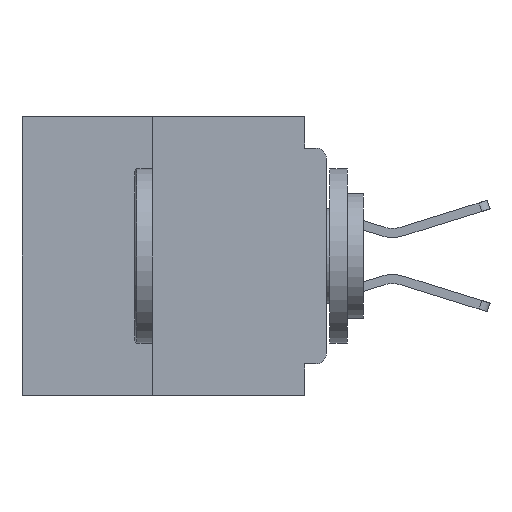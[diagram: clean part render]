
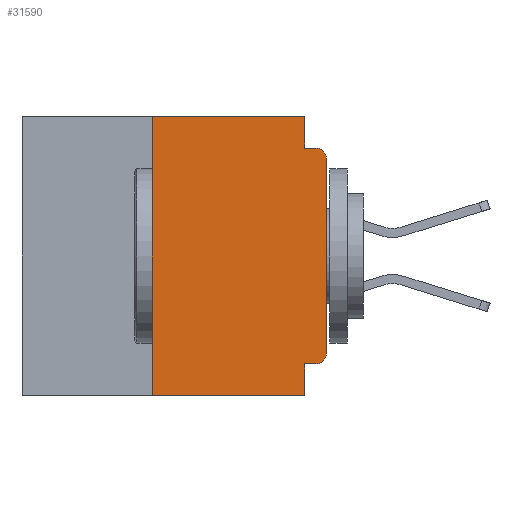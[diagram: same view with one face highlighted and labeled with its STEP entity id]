
A CAD part, left-side view. The second image highlights one B-rep face of the part: STEP entity #31590.
In plain terms, the highlighted planar face has unit normal (-1, 0, 0).
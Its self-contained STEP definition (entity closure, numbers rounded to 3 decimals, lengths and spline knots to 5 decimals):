
#134 = DIRECTION ( 'NONE',  ( 0., 0., -1. ) ) ;
#167 = LINE ( 'NONE', #49163, #48025 ) ;
#2944 = DIRECTION ( 'NONE',  ( 0., 0., -1. ) ) ;
#3805 = DIRECTION ( 'NONE',  ( 0., 0., -1. ) ) ;
#4819 = ORIENTED_EDGE ( 'NONE', *, *, #7803, .T. ) ;
#5775 = CARTESIAN_POINT ( 'NONE',  ( 0., 0., 0. ) ) ;
#5936 = LINE ( 'NONE', #54276, #18625 ) ;
#6459 = CARTESIAN_POINT ( 'NONE',  ( 0., 0., -0.06 ) ) ;
#7596 = VERTEX_POINT ( 'NONE', #22908 ) ;
#7803 = EDGE_CURVE ( 'NONE', #50664, #33889, #31660, .T. ) ;
#8249 = VECTOR ( 'NONE', #53485, 39.37008 ) ;
#10193 = VERTEX_POINT ( 'NONE', #15095 ) ;
#10473 = FACE_OUTER_BOUND ( 'NONE', #39620, .T. ) ;
#10834 = VECTOR ( 'NONE', #36608, 39.37008 ) ;
#14037 = VERTEX_POINT ( 'NONE', #52825 ) ;
#14038 = VECTOR ( 'NONE', #58044, 39.37008 ) ;
#14109 = DIRECTION ( 'NONE',  ( -1., 0., 0. ) ) ;
#14757 = VERTEX_POINT ( 'NONE', #58318 ) ;
#14826 = VERTEX_POINT ( 'NONE', #6459 ) ;
#15095 = CARTESIAN_POINT ( 'NONE',  ( 0., 0.015, -0.045 ) ) ;
#15217 = EDGE_CURVE ( 'NONE', #14826, #10193, #20259, .T. ) ;
#15760 = DIRECTION ( 'NONE',  ( 0., -1., 0. ) ) ;
#18625 = VECTOR ( 'NONE', #35677, 39.37008 ) ;
#20004 = CARTESIAN_POINT ( 'NONE',  ( 0., 0., -0.045 ) ) ;
#20259 = CIRCLE ( 'NONE', #28420, 0.015 ) ;
#20455 = VECTOR ( 'NONE', #44018, 39.37008 ) ;
#20880 = LINE ( 'NONE', #26800, #32079 ) ;
#22908 = CARTESIAN_POINT ( 'NONE',  ( 0., 0.015, -0.355 ) ) ;
#23308 = ORIENTED_EDGE ( 'NONE', *, *, #40323, .F. ) ;
#23654 = EDGE_CURVE ( 'NONE', #7596, #14757, #50395, .T. ) ;
#23836 = ORIENTED_EDGE ( 'NONE', *, *, #23654, .F. ) ;
#25021 = CARTESIAN_POINT ( 'NONE',  ( 0., 0.437, -0.4 ) ) ;
#26439 = DIRECTION ( 'NONE',  ( 1., 0., 0. ) ) ;
#26481 = AXIS2_PLACEMENT_3D ( 'NONE', #40672, #26439, #59667 ) ;
#26796 = LINE ( 'NONE', #20004, #14038 ) ;
#26800 = CARTESIAN_POINT ( 'NONE',  ( 0., 0.031, -0.4 ) ) ;
#26834 = EDGE_CURVE ( 'NONE', #50664, #54660, #5936, .T. ) ;
#27673 = ORIENTED_EDGE ( 'NONE', *, *, #26834, .F. ) ;
#28420 = AXIS2_PLACEMENT_3D ( 'NONE', #42783, #14109, #47535 ) ;
#28517 = AXIS2_PLACEMENT_3D ( 'NONE', #57260, #28807, #134 ) ;
#28807 = DIRECTION ( 'NONE',  ( -1., 0., 0. ) ) ;
#30177 = CARTESIAN_POINT ( 'NONE',  ( 0., 0.031, -0.4 ) ) ;
#31411 = EDGE_CURVE ( 'NONE', #34546, #14826, #58930, .T. ) ;
#31590 = ADVANCED_FACE ( 'NONE', ( #10473 ), #54910, .F. ) ;
#31660 = LINE ( 'NONE', #25021, #20455 ) ;
#31781 = CARTESIAN_POINT ( 'NONE',  ( 0., 0., -0.355 ) ) ;
#32079 = VECTOR ( 'NONE', #2944, 39.37008 ) ;
#32105 = ORIENTED_EDGE ( 'NONE', *, *, #38261, .F. ) ;
#32231 = ORIENTED_EDGE ( 'NONE', *, *, #60220, .T. ) ;
#33188 = CARTESIAN_POINT ( 'NONE',  ( 0., 0., -0.34 ) ) ;
#33889 = VERTEX_POINT ( 'NONE', #30177 ) ;
#34175 = CIRCLE ( 'NONE', #28517, 0.015 ) ;
#34546 = VERTEX_POINT ( 'NONE', #33188 ) ;
#34782 = EDGE_CURVE ( 'NONE', #54660, #14037, #167, .T. ) ;
#35677 = DIRECTION ( 'NONE',  ( 0., 0., 1. ) ) ;
#36435 = ORIENTED_EDGE ( 'NONE', *, *, #31411, .T. ) ;
#36608 = DIRECTION ( 'NONE',  ( 0., 1., 0. ) ) ;
#36715 = ORIENTED_EDGE ( 'NONE', *, *, #34782, .F. ) ;
#37222 = EDGE_CURVE ( 'NONE', #14757, #33889, #20880, .T. ) ;
#38261 = EDGE_CURVE ( 'NONE', #45914, #10193, #26796, .T. ) ;
#38738 = CARTESIAN_POINT ( 'NONE',  ( 0., 0.25, -0.4 ) ) ;
#39620 = EDGE_LOOP ( 'NONE', ( #36435, #57148, #32105, #23308, #36715, #27673, #4819, #41605, #23836, #32231 ) ) ;
#40323 = EDGE_CURVE ( 'NONE', #14037, #45914, #60676, .T. ) ;
#40672 = CARTESIAN_POINT ( 'NONE',  ( 0., 0.437, 0. ) ) ;
#41605 = ORIENTED_EDGE ( 'NONE', *, *, #37222, .F. ) ;
#42783 = CARTESIAN_POINT ( 'NONE',  ( 0., 0.015, -0.06 ) ) ;
#44018 = DIRECTION ( 'NONE',  ( 0., -1., 0. ) ) ;
#45914 = VERTEX_POINT ( 'NONE', #59237 ) ;
#46657 = VECTOR ( 'NONE', #3805, 39.37008 ) ;
#47535 = DIRECTION ( 'NONE',  ( 0., 0., -1. ) ) ;
#48025 = VECTOR ( 'NONE', #15760, 39.37008 ) ;
#49163 = CARTESIAN_POINT ( 'NONE',  ( 0., 0.437, 0. ) ) ;
#50395 = LINE ( 'NONE', #31781, #10834 ) ;
#50664 = VERTEX_POINT ( 'NONE', #38738 ) ;
#51380 = CARTESIAN_POINT ( 'NONE',  ( 0., 0.031, 0. ) ) ;
#52825 = CARTESIAN_POINT ( 'NONE',  ( 0., 0.031, 0. ) ) ;
#53485 = DIRECTION ( 'NONE',  ( 0., 0., 1. ) ) ;
#54276 = CARTESIAN_POINT ( 'NONE',  ( 0., 0.25, -0.4 ) ) ;
#54660 = VERTEX_POINT ( 'NONE', #60538 ) ;
#54910 = PLANE ( 'NONE',  #26481 ) ;
#57148 = ORIENTED_EDGE ( 'NONE', *, *, #15217, .T. ) ;
#57260 = CARTESIAN_POINT ( 'NONE',  ( 0., 0.015, -0.34 ) ) ;
#58044 = DIRECTION ( 'NONE',  ( 0., -1., 0. ) ) ;
#58318 = CARTESIAN_POINT ( 'NONE',  ( 0., 0.031, -0.355 ) ) ;
#58930 = LINE ( 'NONE', #5775, #8249 ) ;
#59237 = CARTESIAN_POINT ( 'NONE',  ( 0., 0.031, -0.045 ) ) ;
#59667 = DIRECTION ( 'NONE',  ( 0., 0., -1. ) ) ;
#60220 = EDGE_CURVE ( 'NONE', #7596, #34546, #34175, .T. ) ;
#60538 = CARTESIAN_POINT ( 'NONE',  ( 0., 0.25, 0. ) ) ;
#60676 = LINE ( 'NONE', #51380, #46657 ) ;
